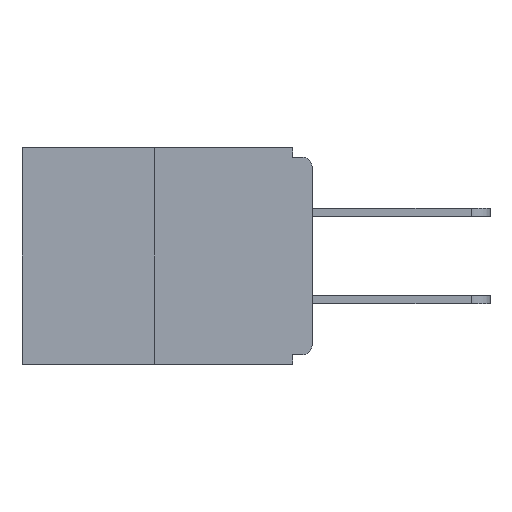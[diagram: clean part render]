
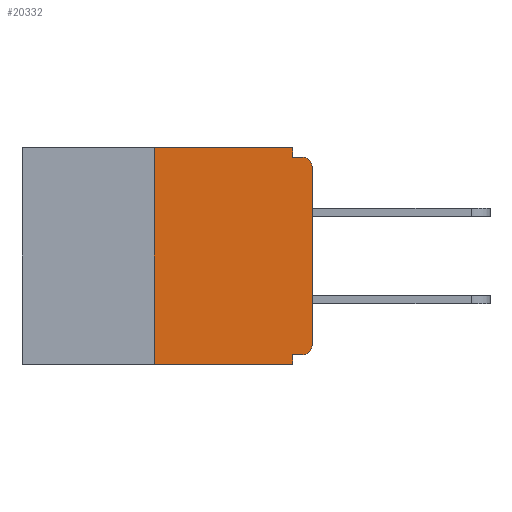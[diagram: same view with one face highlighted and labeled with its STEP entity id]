
A CAD part, left-side view. The second image highlights one B-rep face of the part: STEP entity #20332.
In plain terms, the highlighted planar face has unit normal (-1, 0, 0).
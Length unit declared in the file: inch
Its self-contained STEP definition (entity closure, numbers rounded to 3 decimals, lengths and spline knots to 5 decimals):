
#312 = DIRECTION ( 'NONE',  ( 0., 0., -1. ) ) ;
#509 = LINE ( 'NONE', #8422, #8927 ) ;
#646 = VERTEX_POINT ( 'NONE', #24863 ) ;
#1000 = CARTESIAN_POINT ( 'NONE',  ( 0., 0.031, -0.328 ) ) ;
#1273 = CARTESIAN_POINT ( 'NONE',  ( 0., 0.015, -0.313 ) ) ;
#1914 = CARTESIAN_POINT ( 'NONE',  ( 0., 0.031, 0. ) ) ;
#2552 = CARTESIAN_POINT ( 'NONE',  ( 0., 0.031, 0. ) ) ;
#2705 = EDGE_CURVE ( 'NONE', #646, #12302, #5200, .T. ) ;
#2830 = ORIENTED_EDGE ( 'NONE', *, *, #9289, .T. ) ;
#3020 = CARTESIAN_POINT ( 'NONE',  ( 0., 0.46, 0. ) ) ;
#3371 = VECTOR ( 'NONE', #6986, 39.37008 ) ;
#4254 = CARTESIAN_POINT ( 'NONE',  ( 0., 0.46, 0. ) ) ;
#5136 = DIRECTION ( 'NONE',  ( 0., 0., -1. ) ) ;
#5200 = LINE ( 'NONE', #29221, #29421 ) ;
#5341 = DIRECTION ( 'NONE',  ( -1., 0., 0. ) ) ;
#5795 = ORIENTED_EDGE ( 'NONE', *, *, #22628, .F. ) ;
#6483 = FACE_OUTER_BOUND ( 'NONE', #28000, .T. ) ;
#6890 = CARTESIAN_POINT ( 'NONE',  ( 0., 0., -0.015 ) ) ;
#6986 = DIRECTION ( 'NONE',  ( 0., 1., 0. ) ) ;
#7509 = LINE ( 'NONE', #3020, #29514 ) ;
#7677 = LINE ( 'NONE', #22535, #28283 ) ;
#7879 = VERTEX_POINT ( 'NONE', #28486 ) ;
#7993 = CARTESIAN_POINT ( 'NONE',  ( 0., 0., 0. ) ) ;
#8422 = CARTESIAN_POINT ( 'NONE',  ( 0., 0.25, 0. ) ) ;
#8512 = EDGE_CURVE ( 'NONE', #15328, #12510, #19542, .T. ) ;
#8547 = DIRECTION ( 'NONE',  ( 0., 0., -1. ) ) ;
#8783 = VERTEX_POINT ( 'NONE', #29591 ) ;
#8927 = VECTOR ( 'NONE', #29843, 39.37008 ) ;
#8941 = EDGE_CURVE ( 'NONE', #7879, #24720, #10725, .T. ) ;
#9289 = EDGE_CURVE ( 'NONE', #8783, #10729, #19143, .T. ) ;
#9681 = ORIENTED_EDGE ( 'NONE', *, *, #8941, .F. ) ;
#10326 = EDGE_CURVE ( 'NONE', #12510, #12302, #7677, .T. ) ;
#10400 = AXIS2_PLACEMENT_3D ( 'NONE', #26109, #5341, #5136 ) ;
#10409 = DIRECTION ( 'NONE',  ( 0., 0., -1. ) ) ;
#10725 = LINE ( 'NONE', #6890, #12222 ) ;
#10729 = VERTEX_POINT ( 'NONE', #14520 ) ;
#11885 = DIRECTION ( 'NONE',  ( 1., 0., 0. ) ) ;
#12222 = VECTOR ( 'NONE', #21045, 39.37008 ) ;
#12302 = VERTEX_POINT ( 'NONE', #26155 ) ;
#12386 = EDGE_CURVE ( 'NONE', #23728, #7879, #13875, .T. ) ;
#12414 = VERTEX_POINT ( 'NONE', #26363 ) ;
#12510 = VERTEX_POINT ( 'NONE', #1000 ) ;
#13334 = AXIS2_PLACEMENT_3D ( 'NONE', #1273, #24391, #10409 ) ;
#13875 = LINE ( 'NONE', #2552, #19688 ) ;
#14016 = ORIENTED_EDGE ( 'NONE', *, *, #21760, .T. ) ;
#14520 = CARTESIAN_POINT ( 'NONE',  ( 0., 0., -0.03 ) ) ;
#14811 = AXIS2_PLACEMENT_3D ( 'NONE', #4254, #11885, #21321 ) ;
#15328 = VERTEX_POINT ( 'NONE', #19426 ) ;
#15382 = EDGE_CURVE ( 'NONE', #10729, #24720, #16929, .T. ) ;
#15983 = PLANE ( 'NONE',  #14811 ) ;
#16259 = CARTESIAN_POINT ( 'NONE',  ( 0., 0.015, -0.015 ) ) ;
#16294 = CIRCLE ( 'NONE', #13334, 0.015 ) ;
#16907 = ORIENTED_EDGE ( 'NONE', *, *, #8512, .F. ) ;
#16929 = CIRCLE ( 'NONE', #10400, 0.015 ) ;
#19143 = LINE ( 'NONE', #7993, #29030 ) ;
#19249 = DIRECTION ( 'NONE',  ( 0., -1., 0. ) ) ;
#19426 = CARTESIAN_POINT ( 'NONE',  ( 0., 0.015, -0.328 ) ) ;
#19542 = LINE ( 'NONE', #21482, #3371 ) ;
#19688 = VECTOR ( 'NONE', #312, 39.37008 ) ;
#20332 = ADVANCED_FACE ( 'NONE', ( #6483 ), #15983, .F. ) ;
#21045 = DIRECTION ( 'NONE',  ( 0., -1., 0. ) ) ;
#21321 = DIRECTION ( 'NONE',  ( 0., 0., -1. ) ) ;
#21482 = CARTESIAN_POINT ( 'NONE',  ( 0., 0., -0.328 ) ) ;
#21565 = EDGE_CURVE ( 'NONE', #12414, #23728, #7509, .T. ) ;
#21760 = EDGE_CURVE ( 'NONE', #15328, #8783, #16294, .T. ) ;
#21940 = ORIENTED_EDGE ( 'NONE', *, *, #15382, .T. ) ;
#22535 = CARTESIAN_POINT ( 'NONE',  ( 0., 0.031, -0.343 ) ) ;
#22628 = EDGE_CURVE ( 'NONE', #646, #12414, #509, .T. ) ;
#22973 = ORIENTED_EDGE ( 'NONE', *, *, #21565, .F. ) ;
#23044 = ORIENTED_EDGE ( 'NONE', *, *, #10326, .F. ) ;
#23187 = ORIENTED_EDGE ( 'NONE', *, *, #12386, .F. ) ;
#23728 = VERTEX_POINT ( 'NONE', #1914 ) ;
#24391 = DIRECTION ( 'NONE',  ( -1., 0., 0. ) ) ;
#24720 = VERTEX_POINT ( 'NONE', #16259 ) ;
#24863 = CARTESIAN_POINT ( 'NONE',  ( 0., 0.25, -0.343 ) ) ;
#25088 = ORIENTED_EDGE ( 'NONE', *, *, #2705, .T. ) ;
#26109 = CARTESIAN_POINT ( 'NONE',  ( 0., 0.015, -0.03 ) ) ;
#26155 = CARTESIAN_POINT ( 'NONE',  ( 0., 0.031, -0.343 ) ) ;
#26363 = CARTESIAN_POINT ( 'NONE',  ( 0., 0.25, 0. ) ) ;
#28000 = EDGE_LOOP ( 'NONE', ( #22973, #5795, #25088, #23044, #16907, #14016, #2830, #21940, #9681, #23187 ) ) ;
#28283 = VECTOR ( 'NONE', #8547, 39.37008 ) ;
#28486 = CARTESIAN_POINT ( 'NONE',  ( 0., 0.031, -0.015 ) ) ;
#28703 = DIRECTION ( 'NONE',  ( 0., 0., 1. ) ) ;
#29030 = VECTOR ( 'NONE', #28703, 39.37008 ) ;
#29221 = CARTESIAN_POINT ( 'NONE',  ( 0., 0.46, -0.343 ) ) ;
#29322 = DIRECTION ( 'NONE',  ( 0., -1., 0. ) ) ;
#29421 = VECTOR ( 'NONE', #29322, 39.37008 ) ;
#29514 = VECTOR ( 'NONE', #19249, 39.37008 ) ;
#29591 = CARTESIAN_POINT ( 'NONE',  ( 0., 0., -0.313 ) ) ;
#29843 = DIRECTION ( 'NONE',  ( 0., 0., 1. ) ) ;
